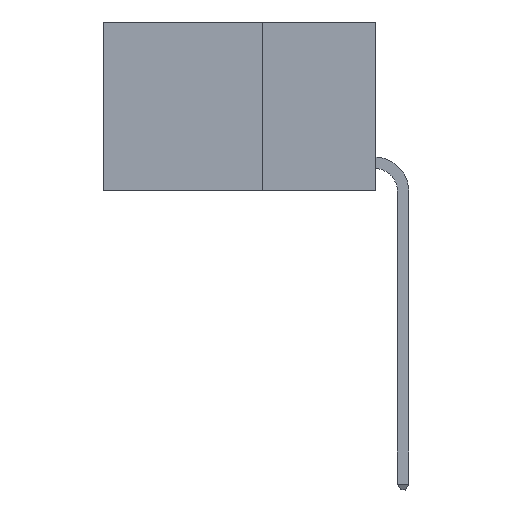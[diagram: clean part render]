
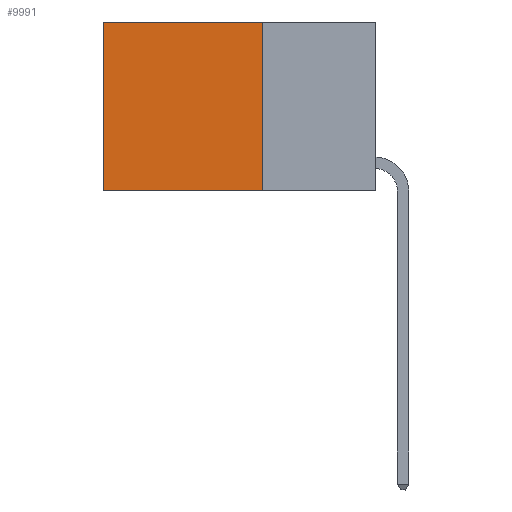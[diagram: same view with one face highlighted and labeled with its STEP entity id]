
A CAD part, left-side view. The second image highlights one B-rep face of the part: STEP entity #9991.
In plain terms, the highlighted planar face has unit normal (-1, 0, 0).
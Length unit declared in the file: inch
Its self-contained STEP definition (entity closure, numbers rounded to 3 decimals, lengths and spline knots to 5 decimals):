
#201 = EDGE_CURVE ( 'NONE', #6159, #12627, #15027, .T. ) ;
#394 = EDGE_CURVE ( 'NONE', #18610, #11549, #4116, .T. ) ;
#658 = CARTESIAN_POINT ( 'NONE',  ( 0.2625, 0.25, -0.37 ) ) ;
#1281 = CARTESIAN_POINT ( 'NONE',  ( 0.2625, 0.25, 0. ) ) ;
#1288 = VECTOR ( 'NONE', #23291, 39.37008 ) ;
#1334 = ORIENTED_EDGE ( 'NONE', *, *, #2096, .T. ) ;
#2096 = EDGE_CURVE ( 'NONE', #12627, #11549, #4842, .T. ) ;
#3028 = AXIS2_PLACEMENT_3D ( 'NONE', #13566, #8862, #6985 ) ;
#4084 = ORIENTED_EDGE ( 'NONE', *, *, #201, .T. ) ;
#4116 = LINE ( 'NONE', #12841, #19898 ) ;
#4842 = LINE ( 'NONE', #8868, #1288 ) ;
#6159 = VERTEX_POINT ( 'NONE', #1281 ) ;
#6958 = DIRECTION ( 'NONE',  ( 0., 1., 0. ) ) ;
#6985 = DIRECTION ( 'NONE',  ( 0., 0., -1. ) ) ;
#7190 = ORIENTED_EDGE ( 'NONE', *, *, #394, .F. ) ;
#8862 = DIRECTION ( 'NONE',  ( 1., 0., 0. ) ) ;
#8868 = CARTESIAN_POINT ( 'NONE',  ( 0.2625, 0.6, 0. ) ) ;
#9339 = CARTESIAN_POINT ( 'NONE',  ( 0.2625, 0.25, 0. ) ) ;
#9991 = ADVANCED_FACE ( 'NONE', ( #17477 ), #15599, .F. ) ;
#11549 = VERTEX_POINT ( 'NONE', #13999 ) ;
#12627 = VERTEX_POINT ( 'NONE', #26060 ) ;
#12841 = CARTESIAN_POINT ( 'NONE',  ( 0.2625, 0.25, -0.37 ) ) ;
#13566 = CARTESIAN_POINT ( 'NONE',  ( 0.2625, 0.25, 0. ) ) ;
#13624 = LINE ( 'NONE', #9339, #14621 ) ;
#13999 = CARTESIAN_POINT ( 'NONE',  ( 0.2625, 0.6, -0.37 ) ) ;
#14563 = EDGE_LOOP ( 'NONE', ( #1334, #7190, #18403, #4084 ) ) ;
#14621 = VECTOR ( 'NONE', #17533, 39.37008 ) ;
#15027 = LINE ( 'NONE', #21648, #25045 ) ;
#15599 = PLANE ( 'NONE',  #3028 ) ;
#16201 = EDGE_CURVE ( 'NONE', #6159, #18610, #13624, .T. ) ;
#17477 = FACE_OUTER_BOUND ( 'NONE', #14563, .T. ) ;
#17533 = DIRECTION ( 'NONE',  ( 0., 0., -1. ) ) ;
#18403 = ORIENTED_EDGE ( 'NONE', *, *, #16201, .F. ) ;
#18610 = VERTEX_POINT ( 'NONE', #658 ) ;
#19898 = VECTOR ( 'NONE', #20661, 39.37008 ) ;
#20661 = DIRECTION ( 'NONE',  ( 0., 1., 0. ) ) ;
#21648 = CARTESIAN_POINT ( 'NONE',  ( 0.2625, 0.25, 0. ) ) ;
#23291 = DIRECTION ( 'NONE',  ( 0., 0., -1. ) ) ;
#25045 = VECTOR ( 'NONE', #6958, 39.37008 ) ;
#26060 = CARTESIAN_POINT ( 'NONE',  ( 0.2625, 0.6, 0. ) ) ;
